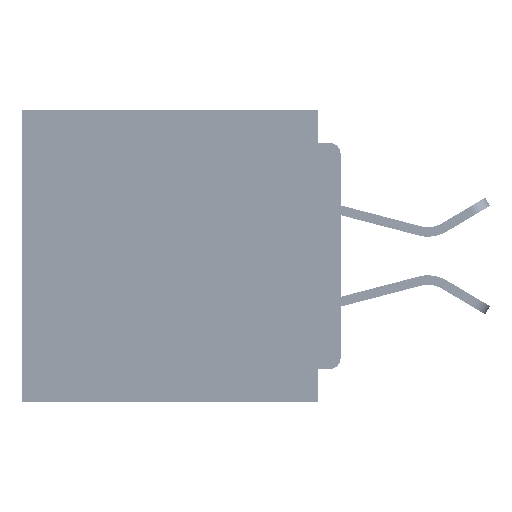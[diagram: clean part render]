
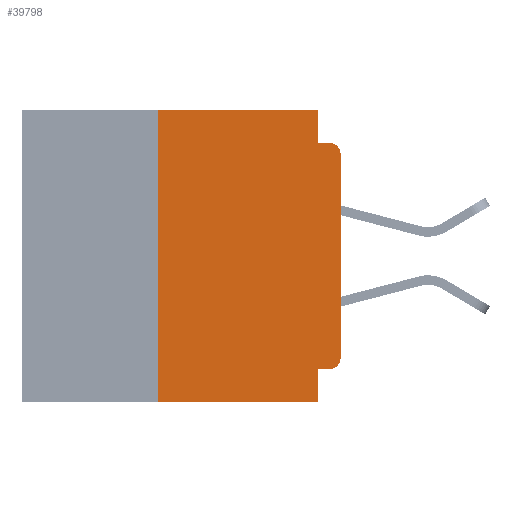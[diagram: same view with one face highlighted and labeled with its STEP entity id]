
A CAD part, left-side view. The second image highlights one B-rep face of the part: STEP entity #39798.
In plain terms, the highlighted planar face has unit normal (-1, 0, 0).
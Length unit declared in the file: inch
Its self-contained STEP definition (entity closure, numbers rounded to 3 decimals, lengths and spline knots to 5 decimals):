
#230 = CARTESIAN_POINT ( 'NONE',  ( 0., 0.015, -0.34 ) ) ;
#373 = DIRECTION ( 'NONE',  ( 0., -1., 0. ) ) ;
#479 = DIRECTION ( 'NONE',  ( 0., 1., 0. ) ) ;
#1500 = ORIENTED_EDGE ( 'NONE', *, *, #18824, .T. ) ;
#1826 = AXIS2_PLACEMENT_3D ( 'NONE', #54023, #14181, #49423 ) ;
#5329 = DIRECTION ( 'NONE',  ( 0., 0., -1. ) ) ;
#5517 = LINE ( 'NONE', #26253, #57522 ) ;
#7885 = ORIENTED_EDGE ( 'NONE', *, *, #43353, .T. ) ;
#9303 = VERTEX_POINT ( 'NONE', #9415 ) ;
#9415 = CARTESIAN_POINT ( 'NONE',  ( 0., 0.25, 0. ) ) ;
#11194 = DIRECTION ( 'NONE',  ( 0., -1., 0. ) ) ;
#11534 = VERTEX_POINT ( 'NONE', #23071 ) ;
#12629 = ORIENTED_EDGE ( 'NONE', *, *, #22390, .F. ) ;
#13266 = VERTEX_POINT ( 'NONE', #51525 ) ;
#13316 = DIRECTION ( 'NONE',  ( 0., 0., 1. ) ) ;
#14075 = DIRECTION ( 'NONE',  ( 0., 0., -1. ) ) ;
#14115 = CARTESIAN_POINT ( 'NONE',  ( 0., 0.015, -0.355 ) ) ;
#14181 = DIRECTION ( 'NONE',  ( 1., 0., 0. ) ) ;
#14224 = ORIENTED_EDGE ( 'NONE', *, *, #14693, .F. ) ;
#14693 = EDGE_CURVE ( 'NONE', #46322, #9303, #58341, .T. ) ;
#17665 = DIRECTION ( 'NONE',  ( -1., 0., 0. ) ) ;
#17906 = CIRCLE ( 'NONE', #60993, 0.015 ) ;
#18185 = FACE_OUTER_BOUND ( 'NONE', #45839, .T. ) ;
#18824 = EDGE_CURVE ( 'NONE', #45379, #24919, #17906, .T. ) ;
#19808 = ORIENTED_EDGE ( 'NONE', *, *, #34103, .F. ) ;
#19870 = VECTOR ( 'NONE', #42039, 39.37008 ) ;
#22219 = VECTOR ( 'NONE', #13316, 39.37008 ) ;
#22390 = EDGE_CURVE ( 'NONE', #9303, #13266, #45098, .T. ) ;
#22568 = EDGE_CURVE ( 'NONE', #45961, #45379, #60781, .T. ) ;
#22893 = DIRECTION ( 'NONE',  ( 0., 0., -1. ) ) ;
#22973 = DIRECTION ( 'NONE',  ( 0., 0., 1. ) ) ;
#23071 = CARTESIAN_POINT ( 'NONE',  ( 0., 0.031, -0.045 ) ) ;
#24919 = VERTEX_POINT ( 'NONE', #26495 ) ;
#26253 = CARTESIAN_POINT ( 'NONE',  ( 0., 0., -0.045 ) ) ;
#26495 = CARTESIAN_POINT ( 'NONE',  ( 0., 0.015, -0.045 ) ) ;
#27480 = VERTEX_POINT ( 'NONE', #14115 ) ;
#27548 = EDGE_CURVE ( 'NONE', #46322, #33760, #58087, .T. ) ;
#27963 = CARTESIAN_POINT ( 'NONE',  ( 0., 0.031, -0.355 ) ) ;
#28412 = ORIENTED_EDGE ( 'NONE', *, *, #47298, .F. ) ;
#28434 = CARTESIAN_POINT ( 'NONE',  ( 0., 0., -0.34 ) ) ;
#28550 = CARTESIAN_POINT ( 'NONE',  ( 0., 0., 0. ) ) ;
#30113 = VECTOR ( 'NONE', #22973, 39.37008 ) ;
#33263 = LINE ( 'NONE', #59173, #45046 ) ;
#33274 = CARTESIAN_POINT ( 'NONE',  ( 0., 0.031, -0.4 ) ) ;
#33738 = VERTEX_POINT ( 'NONE', #27963 ) ;
#33760 = VERTEX_POINT ( 'NONE', #33274 ) ;
#33945 = ORIENTED_EDGE ( 'NONE', *, *, #22568, .T. ) ;
#34103 = EDGE_CURVE ( 'NONE', #27480, #33738, #57201, .T. ) ;
#35647 = DIRECTION ( 'NONE',  ( -1., 0., 0. ) ) ;
#35771 = CARTESIAN_POINT ( 'NONE',  ( 0., 0.437, -0.4 ) ) ;
#39798 = ADVANCED_FACE ( 'NONE', ( #18185 ), #64309, .F. ) ;
#42039 = DIRECTION ( 'NONE',  ( 0., -1., 0. ) ) ;
#43215 = VECTOR ( 'NONE', #373, 39.37008 ) ;
#43353 = EDGE_CURVE ( 'NONE', #27480, #45961, #45484, .T. ) ;
#43888 = VECTOR ( 'NONE', #479, 39.37008 ) ;
#44982 = ORIENTED_EDGE ( 'NONE', *, *, #52832, .F. ) ;
#45046 = VECTOR ( 'NONE', #14075, 39.37008 ) ;
#45098 = LINE ( 'NONE', #62196, #19870 ) ;
#45379 = VERTEX_POINT ( 'NONE', #53772 ) ;
#45484 = CIRCLE ( 'NONE', #51900, 0.015 ) ;
#45839 = EDGE_LOOP ( 'NONE', ( #33945, #1500, #28412, #44982, #12629, #14224, #47382, #55207, #19808, #7885 ) ) ;
#45961 = VERTEX_POINT ( 'NONE', #28434 ) ;
#46322 = VERTEX_POINT ( 'NONE', #46677 ) ;
#46677 = CARTESIAN_POINT ( 'NONE',  ( 0., 0.25, -0.4 ) ) ;
#47298 = EDGE_CURVE ( 'NONE', #11534, #24919, #5517, .T. ) ;
#47382 = ORIENTED_EDGE ( 'NONE', *, *, #27548, .T. ) ;
#47839 = CARTESIAN_POINT ( 'NONE',  ( 0., 0.015, -0.06 ) ) ;
#48087 = CARTESIAN_POINT ( 'NONE',  ( 0., 0.25, -0.4 ) ) ;
#49423 = DIRECTION ( 'NONE',  ( 0., 0., -1. ) ) ;
#51525 = CARTESIAN_POINT ( 'NONE',  ( 0., 0.031, 0. ) ) ;
#51900 = AXIS2_PLACEMENT_3D ( 'NONE', #230, #35647, #5329 ) ;
#52832 = EDGE_CURVE ( 'NONE', #13266, #11534, #33263, .T. ) ;
#52842 = DIRECTION ( 'NONE',  ( 0., 0., -1. ) ) ;
#53015 = CARTESIAN_POINT ( 'NONE',  ( 0., 0.031, -0.4 ) ) ;
#53772 = CARTESIAN_POINT ( 'NONE',  ( 0., 0., -0.06 ) ) ;
#54023 = CARTESIAN_POINT ( 'NONE',  ( 0., 0.437, 0. ) ) ;
#54887 = VECTOR ( 'NONE', #22893, 39.37008 ) ;
#55207 = ORIENTED_EDGE ( 'NONE', *, *, #62483, .F. ) ;
#56427 = LINE ( 'NONE', #53015, #54887 ) ;
#57201 = LINE ( 'NONE', #60888, #43888 ) ;
#57522 = VECTOR ( 'NONE', #11194, 39.37008 ) ;
#58087 = LINE ( 'NONE', #35771, #43215 ) ;
#58341 = LINE ( 'NONE', #48087, #30113 ) ;
#59173 = CARTESIAN_POINT ( 'NONE',  ( 0., 0.031, 0. ) ) ;
#60781 = LINE ( 'NONE', #28550, #22219 ) ;
#60888 = CARTESIAN_POINT ( 'NONE',  ( 0., 0., -0.355 ) ) ;
#60993 = AXIS2_PLACEMENT_3D ( 'NONE', #47839, #17665, #52842 ) ;
#62196 = CARTESIAN_POINT ( 'NONE',  ( 0., 0.437, 0. ) ) ;
#62483 = EDGE_CURVE ( 'NONE', #33738, #33760, #56427, .T. ) ;
#64309 = PLANE ( 'NONE',  #1826 ) ;
